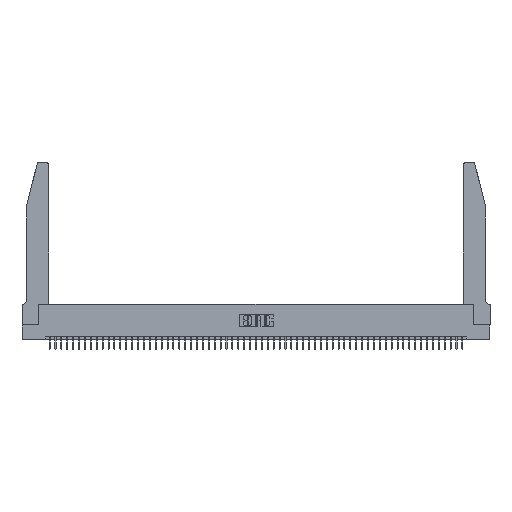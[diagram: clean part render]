
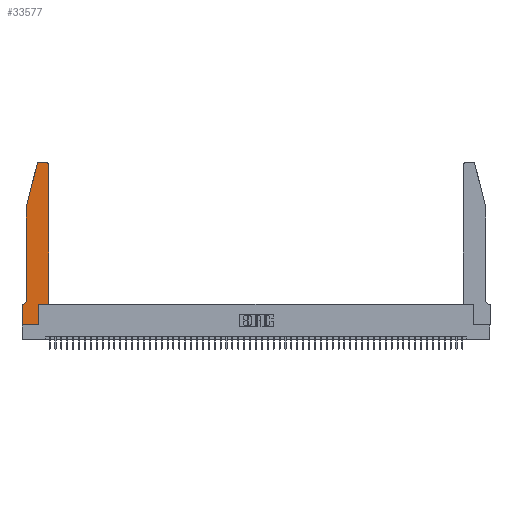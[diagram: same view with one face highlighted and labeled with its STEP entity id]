
A CAD part, top view. The second image highlights one B-rep face of the part: STEP entity #33577.
In plain terms, the highlighted planar face has unit normal (0, 0, 1).
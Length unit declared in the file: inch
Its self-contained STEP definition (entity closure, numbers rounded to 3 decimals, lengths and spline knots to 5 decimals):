
#649 = CARTESIAN_POINT ( 'NONE',  ( 0., 0., 0.37 ) ) ;
#1003 = VERTEX_POINT ( 'NONE', #36309 ) ;
#2948 = FACE_OUTER_BOUND ( 'NONE', #32318, .T. ) ;
#2977 = ORIENTED_EDGE ( 'NONE', *, *, #26101, .T. ) ;
#3674 = CIRCLE ( 'NONE', #49912, 0.07 ) ;
#3846 = EDGE_CURVE ( 'NONE', #54791, #30139, #7562, .T. ) ;
#4258 = ORIENTED_EDGE ( 'NONE', *, *, #35776, .T. ) ;
#4373 = EDGE_CURVE ( 'NONE', #36481, #27184, #49901, .T. ) ;
#4982 = ORIENTED_EDGE ( 'NONE', *, *, #39310, .T. ) ;
#5132 = DIRECTION ( 'NONE',  ( 1., 0., 0. ) ) ;
#6442 = LINE ( 'NONE', #10434, #50186 ) ;
#7562 = LINE ( 'NONE', #31201, #29516 ) ;
#8090 = VECTOR ( 'NONE', #5132, 39.37008 ) ;
#8219 = CARTESIAN_POINT ( 'NONE',  ( 0.2865, 0.35, 0.37 ) ) ;
#8356 = ORIENTED_EDGE ( 'NONE', *, *, #53730, .T. ) ;
#8518 = CARTESIAN_POINT ( 'NONE',  ( 0.4505, 0.35, 0.37 ) ) ;
#8744 = EDGE_CURVE ( 'NONE', #26678, #29253, #14388, .T. ) ;
#9164 = DIRECTION ( 'NONE',  ( 0., 1., 0. ) ) ;
#10434 = CARTESIAN_POINT ( 'NONE',  ( 0.0755, 0.35, 0.37 ) ) ;
#12714 = AXIS2_PLACEMENT_3D ( 'NONE', #48659, #22523, #53016 ) ;
#13103 = EDGE_CURVE ( 'NONE', #44378, #50038, #6442, .T. ) ;
#13762 = DIRECTION ( 'NONE',  ( 0., 0., 1. ) ) ;
#13795 = CARTESIAN_POINT ( 'NONE',  ( 0.4205, 2.75, 0.37 ) ) ;
#14388 = CIRCLE ( 'NONE', #14441, 0.03 ) ;
#14441 = AXIS2_PLACEMENT_3D ( 'NONE', #40001, #13762, #44415 ) ;
#14655 = CARTESIAN_POINT ( 'NONE',  ( 0.0755, 2., 0.37 ) ) ;
#15829 = LINE ( 'NONE', #14655, #37731 ) ;
#16851 = VECTOR ( 'NONE', #26192, 39.37008 ) ;
#17843 = CARTESIAN_POINT ( 'NONE',  ( 0.4505, 2.72, 0.37 ) ) ;
#19555 = CARTESIAN_POINT ( 'NONE',  ( 0., 0., 0.37 ) ) ;
#19813 = VERTEX_POINT ( 'NONE', #21469 ) ;
#20154 = ORIENTED_EDGE ( 'NONE', *, *, #23088, .T. ) ;
#20324 = VECTOR ( 'NONE', #37845, 39.37008 ) ;
#21469 = CARTESIAN_POINT ( 'NONE',  ( 0.2865, 0., 0.37 ) ) ;
#21569 = ORIENTED_EDGE ( 'NONE', *, *, #4373, .T. ) ;
#21609 = DIRECTION ( 'NONE',  ( 0., 0., 1. ) ) ;
#22236 = ORIENTED_EDGE ( 'NONE', *, *, #3846, .T. ) ;
#22333 = PLANE ( 'NONE',  #12714 ) ;
#22485 = CARTESIAN_POINT ( 'NONE',  ( 0.0055, 0.42, 0.37 ) ) ;
#22523 = DIRECTION ( 'NONE',  ( 0., 0., 1. ) ) ;
#22635 = DIRECTION ( 'NONE',  ( 1., 0., 0. ) ) ;
#23088 = EDGE_CURVE ( 'NONE', #19813, #54791, #50738, .T. ) ;
#23990 = DIRECTION ( 'NONE',  ( 0., -1., 0. ) ) ;
#26101 = EDGE_CURVE ( 'NONE', #26963, #19813, #43052, .T. ) ;
#26192 = DIRECTION ( 'NONE',  ( 0., 1., 0. ) ) ;
#26214 = ORIENTED_EDGE ( 'NONE', *, *, #8744, .T. ) ;
#26678 = VERTEX_POINT ( 'NONE', #41045 ) ;
#26893 = DIRECTION ( 'NONE',  ( -1., 0., 0. ) ) ;
#26963 = VERTEX_POINT ( 'NONE', #51479 ) ;
#27184 = VERTEX_POINT ( 'NONE', #13795 ) ;
#27440 = EDGE_CURVE ( 'NONE', #50038, #26963, #53037, .T. ) ;
#27746 = ORIENTED_EDGE ( 'NONE', *, *, #31899, .T. ) ;
#28950 = VECTOR ( 'NONE', #9164, 39.37008 ) ;
#28962 = CARTESIAN_POINT ( 'NONE',  ( 0.25487, 2.72718, 0.37 ) ) ;
#29253 = VERTEX_POINT ( 'NONE', #28962 ) ;
#29516 = VECTOR ( 'NONE', #22635, 39.37008 ) ;
#29714 = CARTESIAN_POINT ( 'NONE',  ( 0.0755, 0.42, 0.37 ) ) ;
#30139 = VERTEX_POINT ( 'NONE', #52080 ) ;
#31014 = CARTESIAN_POINT ( 'NONE',  ( 0.2865, 0.35, 0.37 ) ) ;
#31201 = CARTESIAN_POINT ( 'NONE',  ( 0.4505, 0.35, 0.37 ) ) ;
#31533 = AXIS2_PLACEMENT_3D ( 'NONE', #47783, #21609, #52123 ) ;
#31899 = EDGE_CURVE ( 'NONE', #30139, #36481, #53040, .T. ) ;
#32318 = EDGE_LOOP ( 'NONE', ( #55498, #26214, #4258, #8356, #4982, #44039, #42011, #2977, #20154, #22236, #27746, #21569 ) ) ;
#32464 = DIRECTION ( 'NONE',  ( -1., 0., 0. ) ) ;
#33410 = CARTESIAN_POINT ( 'NONE',  ( 0.2605, 2.75, 0.37 ) ) ;
#33577 = ADVANCED_FACE ( 'NONE', ( #2948 ), #22333, .T. ) ;
#33714 = CARTESIAN_POINT ( 'NONE',  ( 0.0055, 0.35, 0.37 ) ) ;
#35776 = EDGE_CURVE ( 'NONE', #29253, #1003, #38915, .T. ) ;
#36309 = CARTESIAN_POINT ( 'NONE',  ( 0.0755, 2., 0.37 ) ) ;
#36481 = VERTEX_POINT ( 'NONE', #17843 ) ;
#37539 = VECTOR ( 'NONE', #48281, 39.37008 ) ;
#37563 = EDGE_CURVE ( 'NONE', #27184, #26678, #43593, .T. ) ;
#37731 = VECTOR ( 'NONE', #53976, 39.37008 ) ;
#37845 = DIRECTION ( 'NONE',  ( -1., 0., 0. ) ) ;
#38095 = CARTESIAN_POINT ( 'NONE',  ( 0., 0.35, 0.37 ) ) ;
#38915 = LINE ( 'NONE', #52633, #37539 ) ;
#39310 = EDGE_CURVE ( 'NONE', #56513, #44378, #3674, .T. ) ;
#40001 = CARTESIAN_POINT ( 'NONE',  ( 0.284, 2.72, 0.37 ) ) ;
#40125 = VECTOR ( 'NONE', #23990, 39.37008 ) ;
#41045 = CARTESIAN_POINT ( 'NONE',  ( 0.284, 2.75, 0.37 ) ) ;
#42011 = ORIENTED_EDGE ( 'NONE', *, *, #27440, .T. ) ;
#43052 = LINE ( 'NONE', #649, #8090 ) ;
#43593 = LINE ( 'NONE', #33410, #20324 ) ;
#44039 = ORIENTED_EDGE ( 'NONE', *, *, #13103, .T. ) ;
#44378 = VERTEX_POINT ( 'NONE', #33714 ) ;
#44415 = DIRECTION ( 'NONE',  ( 1., 0., 0. ) ) ;
#47783 = CARTESIAN_POINT ( 'NONE',  ( 0.4205, 2.72, 0.37 ) ) ;
#48281 = DIRECTION ( 'NONE',  ( -0.239, -0.971, 0. ) ) ;
#48659 = CARTESIAN_POINT ( 'NONE',  ( 0., 0.35, 0.37 ) ) ;
#49901 = CIRCLE ( 'NONE', #31533, 0.03 ) ;
#49912 = AXIS2_PLACEMENT_3D ( 'NONE', #22485, #52982, #26893 ) ;
#50038 = VERTEX_POINT ( 'NONE', #38095 ) ;
#50186 = VECTOR ( 'NONE', #32464, 39.37008 ) ;
#50738 = LINE ( 'NONE', #31014, #28950 ) ;
#51479 = CARTESIAN_POINT ( 'NONE',  ( 0., 0., 0.37 ) ) ;
#52080 = CARTESIAN_POINT ( 'NONE',  ( 0.4505, 0.35, 0.37 ) ) ;
#52123 = DIRECTION ( 'NONE',  ( 1., 0., 0. ) ) ;
#52633 = CARTESIAN_POINT ( 'NONE',  ( 0.0755, 2., 0.37 ) ) ;
#52982 = DIRECTION ( 'NONE',  ( 0., 0., -1. ) ) ;
#53016 = DIRECTION ( 'NONE',  ( 1., 0., 0. ) ) ;
#53037 = LINE ( 'NONE', #19555, #40125 ) ;
#53040 = LINE ( 'NONE', #8518, #16851 ) ;
#53730 = EDGE_CURVE ( 'NONE', #1003, #56513, #15829, .T. ) ;
#53976 = DIRECTION ( 'NONE',  ( 0., -1., 0. ) ) ;
#54791 = VERTEX_POINT ( 'NONE', #8219 ) ;
#55498 = ORIENTED_EDGE ( 'NONE', *, *, #37563, .T. ) ;
#56513 = VERTEX_POINT ( 'NONE', #29714 ) ;
